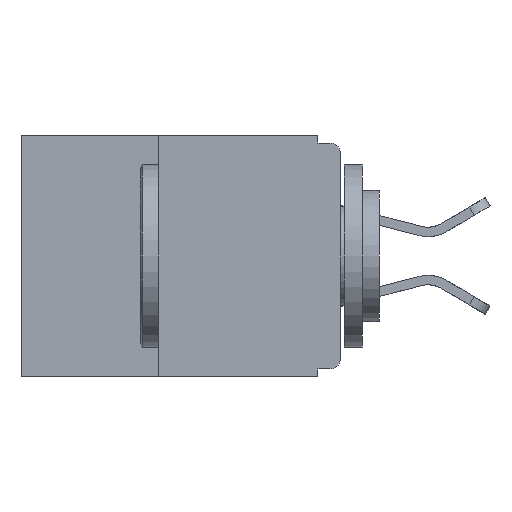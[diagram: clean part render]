
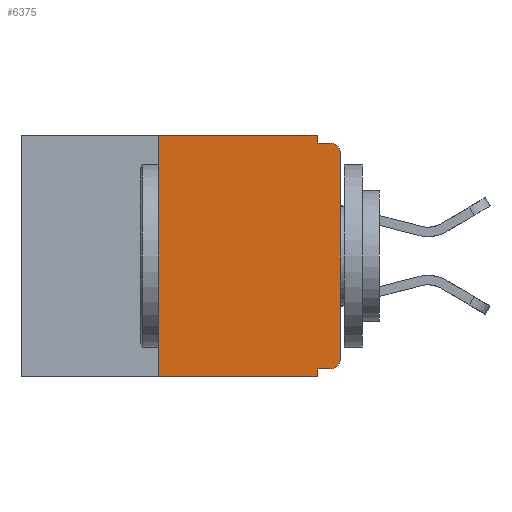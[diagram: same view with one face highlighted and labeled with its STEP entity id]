
A CAD part, left-side view. The second image highlights one B-rep face of the part: STEP entity #6375.
In plain terms, the highlighted planar face has unit normal (-1, 0, 0).
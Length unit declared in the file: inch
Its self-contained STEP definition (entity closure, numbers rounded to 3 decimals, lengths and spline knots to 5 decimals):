
#63 = DIRECTION ( 'NONE',  ( 0., 0., -1. ) ) ;
#485 = LINE ( 'NONE', #7399, #3159 ) ;
#508 = CARTESIAN_POINT ( 'NONE',  ( 0., 0., -0.32 ) ) ;
#935 = VECTOR ( 'NONE', #4024, 39.37008 ) ;
#981 = PLANE ( 'NONE',  #10974 ) ;
#1292 = CIRCLE ( 'NONE', #3419, 0.015 ) ;
#1295 = LINE ( 'NONE', #5848, #935 ) ;
#1390 = CARTESIAN_POINT ( 'NONE',  ( 0., 0.25, 0. ) ) ;
#1549 = ORIENTED_EDGE ( 'NONE', *, *, #3174, .F. ) ;
#1600 = LINE ( 'NONE', #508, #4636 ) ;
#1716 = AXIS2_PLACEMENT_3D ( 'NONE', #1796, #9708, #2931 ) ;
#1796 = CARTESIAN_POINT ( 'NONE',  ( 0., 0.015, -0.305 ) ) ;
#2495 = VERTEX_POINT ( 'NONE', #4133 ) ;
#2529 = ORIENTED_EDGE ( 'NONE', *, *, #8738, .F. ) ;
#2595 = CARTESIAN_POINT ( 'NONE',  ( 0., 0.015, -0.32 ) ) ;
#2725 = ORIENTED_EDGE ( 'NONE', *, *, #8010, .T. ) ;
#2864 = CIRCLE ( 'NONE', #1716, 0.015 ) ;
#2931 = DIRECTION ( 'NONE',  ( 0., 0., -1. ) ) ;
#3080 = EDGE_CURVE ( 'NONE', #8130, #4844, #1295, .T. ) ;
#3119 = DIRECTION ( 'NONE',  ( -1., 0., 0. ) ) ;
#3123 = CARTESIAN_POINT ( 'NONE',  ( 0., 0.25, -0.33 ) ) ;
#3159 = VECTOR ( 'NONE', #12988, 39.37008 ) ;
#3174 = EDGE_CURVE ( 'NONE', #8130, #7801, #9180, .T. ) ;
#3244 = CARTESIAN_POINT ( 'NONE',  ( 0., 0.437, 0. ) ) ;
#3391 = VERTEX_POINT ( 'NONE', #10090 ) ;
#3419 = AXIS2_PLACEMENT_3D ( 'NONE', #9896, #3119, #11019 ) ;
#4003 = DIRECTION ( 'NONE',  ( 0., 0., -1. ) ) ;
#4024 = DIRECTION ( 'NONE',  ( 0., -1., 0. ) ) ;
#4055 = EDGE_CURVE ( 'NONE', #6190, #6278, #12153, .T. ) ;
#4133 = CARTESIAN_POINT ( 'NONE',  ( 0., 0., -0.305 ) ) ;
#4334 = CARTESIAN_POINT ( 'NONE',  ( 0., 0., -0.01 ) ) ;
#4636 = VECTOR ( 'NONE', #5061, 39.37008 ) ;
#4844 = VERTEX_POINT ( 'NONE', #13579 ) ;
#5061 = DIRECTION ( 'NONE',  ( 0., 1., 0. ) ) ;
#5095 = CARTESIAN_POINT ( 'NONE',  ( 0., 0.031, -0.33 ) ) ;
#5363 = EDGE_LOOP ( 'NONE', ( #9372, #12902, #12050, #12976, #6306, #1549, #11052, #9422, #2529, #2725 ) ) ;
#5848 = CARTESIAN_POINT ( 'NONE',  ( 0., 0.437, -0.33 ) ) ;
#6002 = CARTESIAN_POINT ( 'NONE',  ( 0., 0.25, -0.33 ) ) ;
#6190 = VERTEX_POINT ( 'NONE', #11908 ) ;
#6278 = VERTEX_POINT ( 'NONE', #13177 ) ;
#6296 = EDGE_CURVE ( 'NONE', #12206, #3391, #1292, .T. ) ;
#6306 = ORIENTED_EDGE ( 'NONE', *, *, #8987, .F. ) ;
#6375 = ADVANCED_FACE ( 'NONE', ( #11900 ), #981, .F. ) ;
#6684 = DIRECTION ( 'NONE',  ( 0., 0., -1. ) ) ;
#7095 = VECTOR ( 'NONE', #11135, 39.37008 ) ;
#7144 = VERTEX_POINT ( 'NONE', #2595 ) ;
#7399 = CARTESIAN_POINT ( 'NONE',  ( 0., 0., 0. ) ) ;
#7801 = VERTEX_POINT ( 'NONE', #1390 ) ;
#8010 = EDGE_CURVE ( 'NONE', #7144, #2495, #2864, .T. ) ;
#8130 = VERTEX_POINT ( 'NONE', #3123 ) ;
#8152 = CARTESIAN_POINT ( 'NONE',  ( 0., 0.031, 0. ) ) ;
#8546 = CARTESIAN_POINT ( 'NONE',  ( 0., 0., -0.025 ) ) ;
#8563 = LINE ( 'NONE', #4334, #11538 ) ;
#8703 = VECTOR ( 'NONE', #4003, 39.37008 ) ;
#8738 = EDGE_CURVE ( 'NONE', #7144, #9043, #1600, .T. ) ;
#8987 = EDGE_CURVE ( 'NONE', #7801, #6190, #10096, .T. ) ;
#9043 = VERTEX_POINT ( 'NONE', #12367 ) ;
#9180 = LINE ( 'NONE', #6002, #14480 ) ;
#9372 = ORIENTED_EDGE ( 'NONE', *, *, #12776, .T. ) ;
#9422 = ORIENTED_EDGE ( 'NONE', *, *, #11231, .F. ) ;
#9663 = DIRECTION ( 'NONE',  ( 0., 0., 1. ) ) ;
#9708 = DIRECTION ( 'NONE',  ( -1., 0., 0. ) ) ;
#9896 = CARTESIAN_POINT ( 'NONE',  ( 0., 0.015, -0.025 ) ) ;
#10090 = CARTESIAN_POINT ( 'NONE',  ( 0., 0.015, -0.01 ) ) ;
#10096 = LINE ( 'NONE', #3244, #7095 ) ;
#10118 = EDGE_CURVE ( 'NONE', #6278, #3391, #8563, .T. ) ;
#10974 = AXIS2_PLACEMENT_3D ( 'NONE', #13375, #13421, #6684 ) ;
#11019 = DIRECTION ( 'NONE',  ( 0., 0., -1. ) ) ;
#11052 = ORIENTED_EDGE ( 'NONE', *, *, #3080, .T. ) ;
#11068 = DIRECTION ( 'NONE',  ( 0., -1., 0. ) ) ;
#11135 = DIRECTION ( 'NONE',  ( 0., -1., 0. ) ) ;
#11231 = EDGE_CURVE ( 'NONE', #9043, #4844, #12388, .T. ) ;
#11448 = VECTOR ( 'NONE', #63, 39.37008 ) ;
#11538 = VECTOR ( 'NONE', #11068, 39.37008 ) ;
#11900 = FACE_OUTER_BOUND ( 'NONE', #5363, .T. ) ;
#11908 = CARTESIAN_POINT ( 'NONE',  ( 0., 0.031, 0. ) ) ;
#12050 = ORIENTED_EDGE ( 'NONE', *, *, #10118, .F. ) ;
#12153 = LINE ( 'NONE', #8152, #11448 ) ;
#12206 = VERTEX_POINT ( 'NONE', #8546 ) ;
#12367 = CARTESIAN_POINT ( 'NONE',  ( 0., 0.031, -0.32 ) ) ;
#12388 = LINE ( 'NONE', #5095, #8703 ) ;
#12776 = EDGE_CURVE ( 'NONE', #2495, #12206, #485, .T. ) ;
#12902 = ORIENTED_EDGE ( 'NONE', *, *, #6296, .T. ) ;
#12976 = ORIENTED_EDGE ( 'NONE', *, *, #4055, .F. ) ;
#12988 = DIRECTION ( 'NONE',  ( 0., 0., 1. ) ) ;
#13177 = CARTESIAN_POINT ( 'NONE',  ( 0., 0.031, -0.01 ) ) ;
#13375 = CARTESIAN_POINT ( 'NONE',  ( 0., 0.437, 0. ) ) ;
#13421 = DIRECTION ( 'NONE',  ( 1., 0., 0. ) ) ;
#13579 = CARTESIAN_POINT ( 'NONE',  ( 0., 0.031, -0.33 ) ) ;
#14480 = VECTOR ( 'NONE', #9663, 39.37008 ) ;
